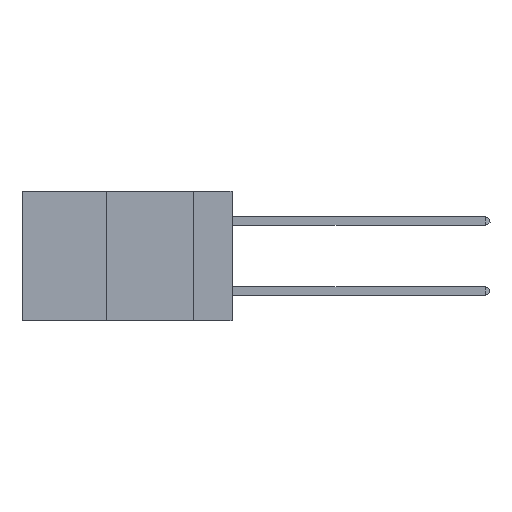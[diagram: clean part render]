
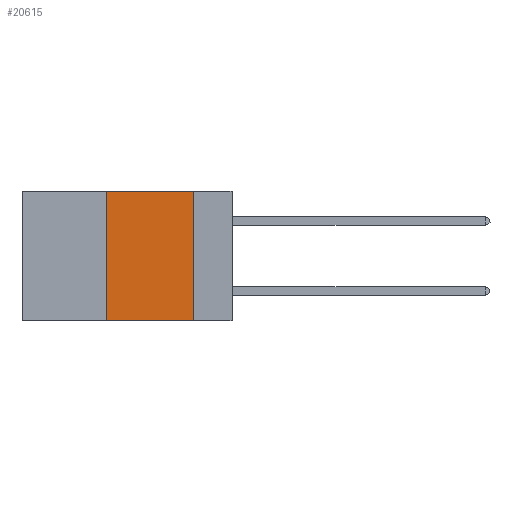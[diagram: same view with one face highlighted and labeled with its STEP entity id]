
A CAD part, left-side view. The second image highlights one B-rep face of the part: STEP entity #20615.
In plain terms, the highlighted planar face has unit normal (-1, 0, 0).
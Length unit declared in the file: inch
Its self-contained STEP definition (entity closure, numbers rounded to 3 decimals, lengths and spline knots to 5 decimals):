
#264 = FACE_OUTER_BOUND ( 'NONE', #14629, .T. ) ;
#314 = VERTEX_POINT ( 'NONE', #13041 ) ;
#318 = DIRECTION ( 'NONE',  ( 0., 0., 1. ) ) ;
#543 = VECTOR ( 'NONE', #9573, 39.37008 ) ;
#1145 = VECTOR ( 'NONE', #318, 39.37008 ) ;
#1976 = CARTESIAN_POINT ( 'NONE',  ( 0., 0.11, -0.37 ) ) ;
#2770 = VERTEX_POINT ( 'NONE', #1976 ) ;
#3347 = VERTEX_POINT ( 'NONE', #3945 ) ;
#3652 = ORIENTED_EDGE ( 'NONE', *, *, #22408, .F. ) ;
#3945 = CARTESIAN_POINT ( 'NONE',  ( 0., 0.11, 0. ) ) ;
#4103 = EDGE_CURVE ( 'NONE', #9311, #3347, #14388, .T. ) ;
#5040 = DIRECTION ( 'NONE',  ( 0., 0., -1. ) ) ;
#6007 = LINE ( 'NONE', #14747, #543 ) ;
#6370 = LINE ( 'NONE', #8953, #1145 ) ;
#6991 = PLANE ( 'NONE',  #16063 ) ;
#8953 = CARTESIAN_POINT ( 'NONE',  ( 0., 0.36, 0. ) ) ;
#9311 = VERTEX_POINT ( 'NONE', #11549 ) ;
#9573 = DIRECTION ( 'NONE',  ( 0., -1., 0. ) ) ;
#10107 = DIRECTION ( 'NONE',  ( 0., 0., -1. ) ) ;
#11549 = CARTESIAN_POINT ( 'NONE',  ( 0., 0.36, 0. ) ) ;
#12219 = LINE ( 'NONE', #17284, #14113 ) ;
#13041 = CARTESIAN_POINT ( 'NONE',  ( 0., 0.36, -0.37 ) ) ;
#13087 = EDGE_CURVE ( 'NONE', #314, #9311, #6370, .T. ) ;
#13666 = CARTESIAN_POINT ( 'NONE',  ( 0., 0.6, 0. ) ) ;
#14113 = VECTOR ( 'NONE', #5040, 39.37008 ) ;
#14207 = ORIENTED_EDGE ( 'NONE', *, *, #20259, .T. ) ;
#14388 = LINE ( 'NONE', #19268, #15478 ) ;
#14629 = EDGE_LOOP ( 'NONE', ( #3652, #16379, #21453, #14207 ) ) ;
#14747 = CARTESIAN_POINT ( 'NONE',  ( 0., 0.6, -0.37 ) ) ;
#15478 = VECTOR ( 'NONE', #21325, 39.37008 ) ;
#16063 = AXIS2_PLACEMENT_3D ( 'NONE', #13666, #20465, #10107 ) ;
#16379 = ORIENTED_EDGE ( 'NONE', *, *, #4103, .F. ) ;
#17284 = CARTESIAN_POINT ( 'NONE',  ( 0., 0.11, 0. ) ) ;
#19268 = CARTESIAN_POINT ( 'NONE',  ( 0., 0.6, 0. ) ) ;
#20259 = EDGE_CURVE ( 'NONE', #314, #2770, #6007, .T. ) ;
#20465 = DIRECTION ( 'NONE',  ( 1., 0., 0. ) ) ;
#20615 = ADVANCED_FACE ( 'NONE', ( #264 ), #6991, .F. ) ;
#21325 = DIRECTION ( 'NONE',  ( 0., -1., 0. ) ) ;
#21453 = ORIENTED_EDGE ( 'NONE', *, *, #13087, .F. ) ;
#22408 = EDGE_CURVE ( 'NONE', #3347, #2770, #12219, .T. ) ;
